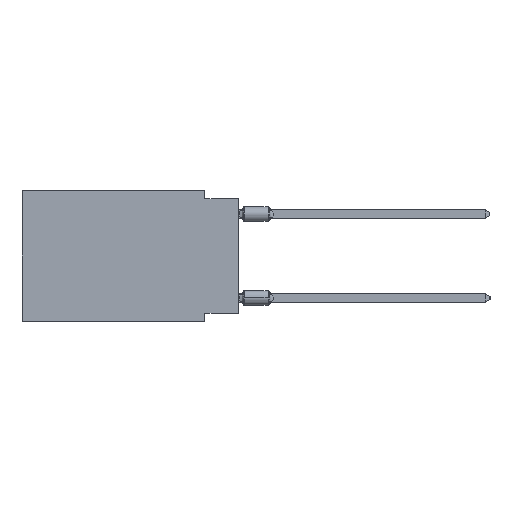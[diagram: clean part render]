
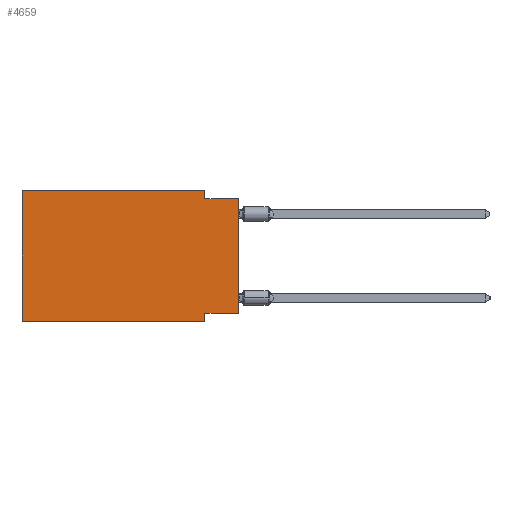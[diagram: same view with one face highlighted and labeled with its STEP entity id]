
A CAD part, left-side view. The second image highlights one B-rep face of the part: STEP entity #4659.
In plain terms, the highlighted planar face has unit normal (-1, 0, 0).
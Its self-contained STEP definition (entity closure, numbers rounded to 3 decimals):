
#1027 = CARTESIAN_POINT ( 'NONE',  ( 0., 16.383, 0. ) ) ;
#1901 = DIRECTION ( 'NONE',  ( 0., 0., -1. ) ) ;
#2572 = ORIENTED_EDGE ( 'NONE', *, *, #25957, .T. ) ;
#3687 = DIRECTION ( 'NONE',  ( 0., -1., 0. ) ) ;
#4659 = ADVANCED_FACE ( 'NONE', ( #10951 ), #24092, .F. ) ;
#4713 = VERTEX_POINT ( 'NONE', #56269 ) ;
#5941 = VERTEX_POINT ( 'NONE', #44984 ) ;
#6225 = ORIENTED_EDGE ( 'NONE', *, *, #33396, .T. ) ;
#6414 = VECTOR ( 'NONE', #3687, 1000. ) ;
#6618 = AXIS2_PLACEMENT_3D ( 'NONE', #1027, #41961, #1901 ) ;
#6980 = VERTEX_POINT ( 'NONE', #34042 ) ;
#7026 = VECTOR ( 'NONE', #53105, 1000. ) ;
#7821 = VERTEX_POINT ( 'NONE', #41240 ) ;
#8915 = CARTESIAN_POINT ( 'NONE',  ( 0., 2.54, -9.271 ) ) ;
#9313 = VERTEX_POINT ( 'NONE', #9586 ) ;
#9352 = VECTOR ( 'NONE', #38768, 1000. ) ;
#9586 = CARTESIAN_POINT ( 'NONE',  ( 0., 2.54, -0.635 ) ) ;
#9779 = VECTOR ( 'NONE', #32251, 1000. ) ;
#10907 = ORIENTED_EDGE ( 'NONE', *, *, #33054, .F. ) ;
#10951 = FACE_OUTER_BOUND ( 'NONE', #11153, .T. ) ;
#11153 = EDGE_LOOP ( 'NONE', ( #2572, #14066, #27145, #10907, #17732, #6225, #49342, #56013 ) ) ;
#11368 = VECTOR ( 'NONE', #53333, 1000. ) ;
#11899 = CARTESIAN_POINT ( 'NONE',  ( 0., 0., 0. ) ) ;
#12470 = LINE ( 'NONE', #11899, #38503 ) ;
#13547 = LINE ( 'NONE', #40169, #9779 ) ;
#14066 = ORIENTED_EDGE ( 'NONE', *, *, #43449, .F. ) ;
#17732 = ORIENTED_EDGE ( 'NONE', *, *, #50694, .F. ) ;
#21526 = DIRECTION ( 'NONE',  ( 0., 0., 1. ) ) ;
#21822 = CARTESIAN_POINT ( 'NONE',  ( 0., 2.54, -9.906 ) ) ;
#24092 = PLANE ( 'NONE',  #6618 ) ;
#25957 = EDGE_CURVE ( 'NONE', #7821, #41704, #12470, .T. ) ;
#26976 = LINE ( 'NONE', #52461, #11368 ) ;
#27145 = ORIENTED_EDGE ( 'NONE', *, *, #39390, .F. ) ;
#30296 = LINE ( 'NONE', #48159, #7026 ) ;
#30638 = CARTESIAN_POINT ( 'NONE',  ( 0., 16.383, 0. ) ) ;
#32251 = DIRECTION ( 'NONE',  ( 0., 0., -1. ) ) ;
#33054 = EDGE_CURVE ( 'NONE', #6980, #4713, #39141, .T. ) ;
#33396 = EDGE_CURVE ( 'NONE', #5941, #46006, #52239, .T. ) ;
#33508 = LINE ( 'NONE', #33804, #48026 ) ;
#33804 = CARTESIAN_POINT ( 'NONE',  ( 0., 0., -9.271 ) ) ;
#34042 = CARTESIAN_POINT ( 'NONE',  ( 0., 16.383, 0. ) ) ;
#34521 = VECTOR ( 'NONE', #39436, 1000. ) ;
#37623 = EDGE_CURVE ( 'NONE', #48892, #46006, #13547, .T. ) ;
#38503 = VECTOR ( 'NONE', #21526, 1000. ) ;
#38768 = DIRECTION ( 'NONE',  ( 0., 0., 1. ) ) ;
#39141 = LINE ( 'NONE', #30638, #34521 ) ;
#39390 = EDGE_CURVE ( 'NONE', #4713, #9313, #30296, .T. ) ;
#39436 = DIRECTION ( 'NONE',  ( 0., -1., 0. ) ) ;
#40169 = CARTESIAN_POINT ( 'NONE',  ( 0., 2.54, -9.906 ) ) ;
#41240 = CARTESIAN_POINT ( 'NONE',  ( 0., 0., -9.271 ) ) ;
#41704 = VERTEX_POINT ( 'NONE', #45922 ) ;
#41961 = DIRECTION ( 'NONE',  ( 1., 0., 0. ) ) ;
#43449 = EDGE_CURVE ( 'NONE', #9313, #41704, #26976, .T. ) ;
#43751 = CARTESIAN_POINT ( 'NONE',  ( 0., 16.383, -9.906 ) ) ;
#44984 = CARTESIAN_POINT ( 'NONE',  ( 0., 16.383, -9.906 ) ) ;
#45922 = CARTESIAN_POINT ( 'NONE',  ( 0., 0., -0.635 ) ) ;
#46006 = VERTEX_POINT ( 'NONE', #21822 ) ;
#46763 = LINE ( 'NONE', #57172, #9352 ) ;
#47691 = EDGE_CURVE ( 'NONE', #7821, #48892, #33508, .T. ) ;
#48026 = VECTOR ( 'NONE', #51367, 1000. ) ;
#48159 = CARTESIAN_POINT ( 'NONE',  ( 0., 2.54, 0. ) ) ;
#48892 = VERTEX_POINT ( 'NONE', #8915 ) ;
#49342 = ORIENTED_EDGE ( 'NONE', *, *, #37623, .F. ) ;
#50694 = EDGE_CURVE ( 'NONE', #5941, #6980, #46763, .T. ) ;
#51367 = DIRECTION ( 'NONE',  ( 0., 1., 0. ) ) ;
#52239 = LINE ( 'NONE', #43751, #6414 ) ;
#52461 = CARTESIAN_POINT ( 'NONE',  ( 0., 0., -0.635 ) ) ;
#53105 = DIRECTION ( 'NONE',  ( 0., 0., -1. ) ) ;
#53333 = DIRECTION ( 'NONE',  ( 0., -1., 0. ) ) ;
#56013 = ORIENTED_EDGE ( 'NONE', *, *, #47691, .F. ) ;
#56269 = CARTESIAN_POINT ( 'NONE',  ( 0., 2.54, 0. ) ) ;
#57172 = CARTESIAN_POINT ( 'NONE',  ( 0., 16.383, 0. ) ) ;
